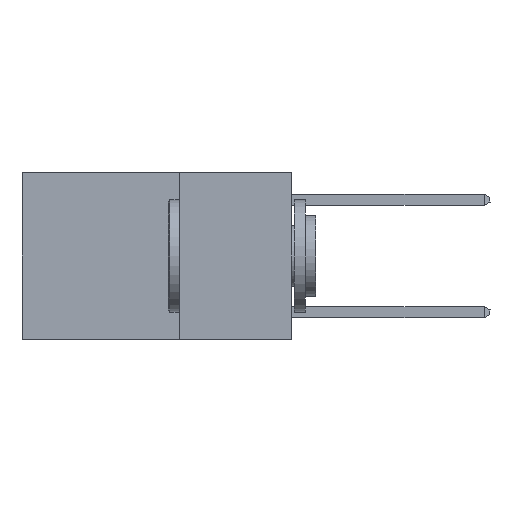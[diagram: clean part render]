
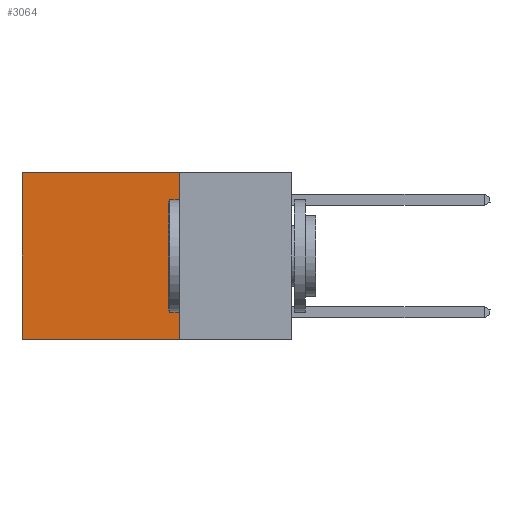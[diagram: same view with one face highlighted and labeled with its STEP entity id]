
A CAD part, left-side view. The second image highlights one B-rep face of the part: STEP entity #3064.
In plain terms, the highlighted planar face has unit normal (-1, 0, 0).
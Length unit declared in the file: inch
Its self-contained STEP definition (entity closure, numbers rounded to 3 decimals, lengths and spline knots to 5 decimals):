
#591 = VERTEX_POINT ( 'NONE', #1382 ) ;
#757 = VERTEX_POINT ( 'NONE', #4014 ) ;
#848 = EDGE_CURVE ( 'NONE', #757, #4487, #7215, .T. ) ;
#964 = LINE ( 'NONE', #2937, #4712 ) ;
#1253 = AXIS2_PLACEMENT_3D ( 'NONE', #2364, #3295, #9792 ) ;
#1382 = CARTESIAN_POINT ( 'NONE',  ( 0.2625, 0.25, 0. ) ) ;
#1513 = CARTESIAN_POINT ( 'NONE',  ( 0.2625, 0.6, 0. ) ) ;
#1628 = ORIENTED_EDGE ( 'NONE', *, *, #6237, .F. ) ;
#1815 = EDGE_CURVE ( 'NONE', #11467, #4487, #964, .T. ) ;
#2091 = DIRECTION ( 'NONE',  ( 0., 0., -1. ) ) ;
#2364 = CARTESIAN_POINT ( 'NONE',  ( 0.2625, 0.25, 0. ) ) ;
#2660 = CARTESIAN_POINT ( 'NONE',  ( 0.2625, 0.25, 0. ) ) ;
#2937 = CARTESIAN_POINT ( 'NONE',  ( 0.2625, 0.6, 0. ) ) ;
#2962 = FACE_OUTER_BOUND ( 'NONE', #4388, .T. ) ;
#3064 = ADVANCED_FACE ( 'NONE', ( #2962 ), #7121, .F. ) ;
#3295 = DIRECTION ( 'NONE',  ( 1., 0., 0. ) ) ;
#3351 = CARTESIAN_POINT ( 'NONE',  ( 0.2625, 0.25, 0. ) ) ;
#4014 = CARTESIAN_POINT ( 'NONE',  ( 0.2625, 0.25, -0.37 ) ) ;
#4388 = EDGE_LOOP ( 'NONE', ( #10476, #9107, #1628, #8751 ) ) ;
#4487 = VERTEX_POINT ( 'NONE', #12028 ) ;
#4667 = VECTOR ( 'NONE', #5491, 39.37008 ) ;
#4712 = VECTOR ( 'NONE', #2091, 39.37008 ) ;
#5267 = LINE ( 'NONE', #3351, #9788 ) ;
#5410 = CARTESIAN_POINT ( 'NONE',  ( 0.2625, 0.25, -0.37 ) ) ;
#5491 = DIRECTION ( 'NONE',  ( 0., 0., -1. ) ) ;
#5828 = LINE ( 'NONE', #2660, #4667 ) ;
#6181 = DIRECTION ( 'NONE',  ( 0., 1., 0. ) ) ;
#6237 = EDGE_CURVE ( 'NONE', #591, #757, #5828, .T. ) ;
#7121 = PLANE ( 'NONE',  #1253 ) ;
#7215 = LINE ( 'NONE', #5410, #10275 ) ;
#8751 = ORIENTED_EDGE ( 'NONE', *, *, #10442, .T. ) ;
#9107 = ORIENTED_EDGE ( 'NONE', *, *, #848, .F. ) ;
#9788 = VECTOR ( 'NONE', #6181, 39.37008 ) ;
#9792 = DIRECTION ( 'NONE',  ( 0., 0., -1. ) ) ;
#10275 = VECTOR ( 'NONE', #11939, 39.37008 ) ;
#10442 = EDGE_CURVE ( 'NONE', #591, #11467, #5267, .T. ) ;
#10476 = ORIENTED_EDGE ( 'NONE', *, *, #1815, .T. ) ;
#11467 = VERTEX_POINT ( 'NONE', #1513 ) ;
#11939 = DIRECTION ( 'NONE',  ( 0., 1., 0. ) ) ;
#12028 = CARTESIAN_POINT ( 'NONE',  ( 0.2625, 0.6, -0.37 ) ) ;
